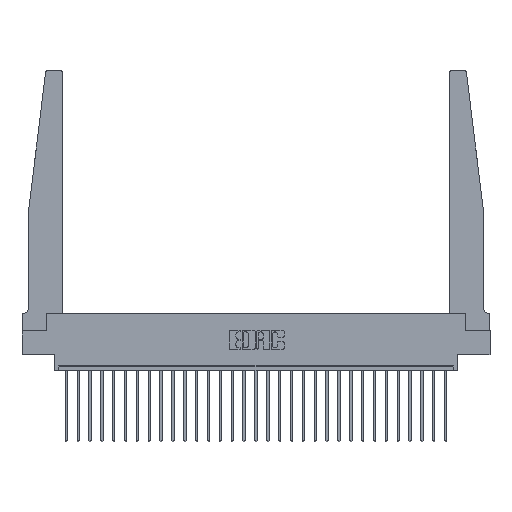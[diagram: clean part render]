
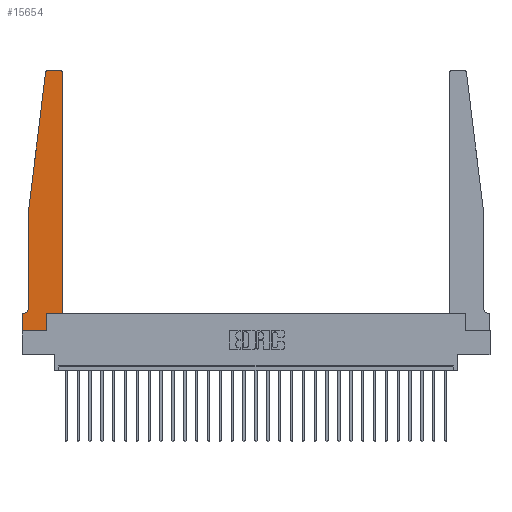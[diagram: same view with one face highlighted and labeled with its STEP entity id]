
A CAD part, top view. The second image highlights one B-rep face of the part: STEP entity #15654.
In plain terms, the highlighted planar face has unit normal (0, 0, 1).
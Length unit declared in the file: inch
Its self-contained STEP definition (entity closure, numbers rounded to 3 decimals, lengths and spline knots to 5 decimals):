
#94 = PLANE ( 'NONE',  #24417 ) ;
#409 = EDGE_CURVE ( 'NONE', #18745, #23858, #8592, .T. ) ;
#501 = FACE_OUTER_BOUND ( 'NONE', #9864, .T. ) ;
#542 = DIRECTION ( 'NONE',  ( 0., -1., 0. ) ) ;
#638 = DIRECTION ( 'NONE',  ( 0., 0., 1. ) ) ;
#757 = DIRECTION ( 'NONE',  ( 1., 0., 0. ) ) ;
#871 = ORIENTED_EDGE ( 'NONE', *, *, #1963, .T. ) ;
#1833 = CARTESIAN_POINT ( 'NONE',  ( 0.065, 1.25, 0.37 ) ) ;
#1963 = EDGE_CURVE ( 'NONE', #26118, #13736, #11295, .T. ) ;
#2018 = EDGE_CURVE ( 'NONE', #22746, #6030, #4937, .T. ) ;
#2330 = LINE ( 'NONE', #15729, #26137 ) ;
#2404 = CARTESIAN_POINT ( 'NONE',  ( 0.2605, 0., 0.37 ) ) ;
#2474 = VERTEX_POINT ( 'NONE', #15890 ) ;
#3025 = VECTOR ( 'NONE', #5932, 39.37008 ) ;
#3362 = DIRECTION ( 'NONE',  ( 0., -1., 0. ) ) ;
#3741 = LINE ( 'NONE', #1833, #3025 ) ;
#4173 = EDGE_CURVE ( 'NONE', #18640, #22746, #21255, .T. ) ;
#4175 = VECTOR ( 'NONE', #26727, 39.37008 ) ;
#4260 = CARTESIAN_POINT ( 'NONE',  ( 0., 0., 0.37 ) ) ;
#4937 = CIRCLE ( 'NONE', #12802, 0.03 ) ;
#5266 = CARTESIAN_POINT ( 'NONE',  ( 0.2605, 0.18, 0.37 ) ) ;
#5402 = DIRECTION ( 'NONE',  ( 0., 0., 1. ) ) ;
#5540 = CARTESIAN_POINT ( 'NONE',  ( 0.27653, 2.75, 0.37 ) ) ;
#5932 = DIRECTION ( 'NONE',  ( -0.122, -0.992, 0. ) ) ;
#6030 = VERTEX_POINT ( 'NONE', #24478 ) ;
#6994 = EDGE_CURVE ( 'NONE', #23858, #26118, #21126, .T. ) ;
#7120 = ORIENTED_EDGE ( 'NONE', *, *, #4173, .T. ) ;
#7160 = ORIENTED_EDGE ( 'NONE', *, *, #13693, .T. ) ;
#7678 = VERTEX_POINT ( 'NONE', #20945 ) ;
#8154 = CARTESIAN_POINT ( 'NONE',  ( 0., 0.1875, 0.37 ) ) ;
#8449 = VERTEX_POINT ( 'NONE', #23913 ) ;
#8592 = LINE ( 'NONE', #10913, #20024 ) ;
#8772 = VECTOR ( 'NONE', #15889, 39.37008 ) ;
#9738 = EDGE_CURVE ( 'NONE', #6030, #22397, #13886, .T. ) ;
#9827 = ORIENTED_EDGE ( 'NONE', *, *, #2018, .T. ) ;
#9864 = EDGE_LOOP ( 'NONE', ( #15268, #23553, #20595, #22302, #7160, #11488, #15987, #17812, #871, #10777, #7120, #9827 ) ) ;
#10184 = EDGE_CURVE ( 'NONE', #22397, #17211, #15628, .T. ) ;
#10320 = VECTOR ( 'NONE', #13755, 39.37008 ) ;
#10777 = ORIENTED_EDGE ( 'NONE', *, *, #18175, .T. ) ;
#10913 = CARTESIAN_POINT ( 'NONE',  ( 0., 0., 0.37 ) ) ;
#10933 = EDGE_CURVE ( 'NONE', #8449, #18745, #2330, .T. ) ;
#11295 = LINE ( 'NONE', #5266, #21563 ) ;
#11404 = DIRECTION ( 'NONE',  ( 0., 0., 1. ) ) ;
#11488 = ORIENTED_EDGE ( 'NONE', *, *, #10933, .T. ) ;
#11969 = LINE ( 'NONE', #18025, #13294 ) ;
#12431 = CARTESIAN_POINT ( 'NONE',  ( 0.015, 0.2375, 0.37 ) ) ;
#12802 = AXIS2_PLACEMENT_3D ( 'NONE', #26090, #5402, #15284 ) ;
#12841 = CARTESIAN_POINT ( 'NONE',  ( 0.2605, 0.18, 0.37 ) ) ;
#13294 = VECTOR ( 'NONE', #3362, 39.37008 ) ;
#13361 = CARTESIAN_POINT ( 'NONE',  ( 0.25, 2.75, 0.37 ) ) ;
#13609 = CARTESIAN_POINT ( 'NONE',  ( 0.24675, 2.72367, 0.37 ) ) ;
#13693 = EDGE_CURVE ( 'NONE', #2474, #8449, #18365, .T. ) ;
#13736 = VERTEX_POINT ( 'NONE', #12841 ) ;
#13755 = DIRECTION ( 'NONE',  ( -1., 0., 0. ) ) ;
#13886 = LINE ( 'NONE', #13361, #10320 ) ;
#14739 = CARTESIAN_POINT ( 'NONE',  ( 0.425, 0.18, 0.37 ) ) ;
#15268 = ORIENTED_EDGE ( 'NONE', *, *, #9738, .T. ) ;
#15284 = DIRECTION ( 'NONE',  ( 1., 0., 0. ) ) ;
#15398 = CARTESIAN_POINT ( 'NONE',  ( 0.27653, 2.72, 0.37 ) ) ;
#15628 = CIRCLE ( 'NONE', #22170, 0.03 ) ;
#15654 = ADVANCED_FACE ( 'NONE', ( #501 ), #94, .T. ) ;
#15729 = CARTESIAN_POINT ( 'NONE',  ( 0.065, 0.1875, 0.37 ) ) ;
#15889 = DIRECTION ( 'NONE',  ( 1., 0., 0. ) ) ;
#15890 = CARTESIAN_POINT ( 'NONE',  ( 0.065, 0.2375, 0.37 ) ) ;
#15959 = EDGE_CURVE ( 'NONE', #17211, #7678, #3741, .T. ) ;
#15987 = ORIENTED_EDGE ( 'NONE', *, *, #409, .T. ) ;
#16226 = CARTESIAN_POINT ( 'NONE',  ( 0.425, 0.18, 0.37 ) ) ;
#16922 = DIRECTION ( 'NONE',  ( 1., 0., 0. ) ) ;
#17211 = VERTEX_POINT ( 'NONE', #13609 ) ;
#17701 = CARTESIAN_POINT ( 'NONE',  ( 0., 0., 0.37 ) ) ;
#17812 = ORIENTED_EDGE ( 'NONE', *, *, #6994, .T. ) ;
#18025 = CARTESIAN_POINT ( 'NONE',  ( 0.065, 1.25, 0.37 ) ) ;
#18175 = EDGE_CURVE ( 'NONE', #13736, #18640, #26285, .T. ) ;
#18258 = CARTESIAN_POINT ( 'NONE',  ( 0.425, 2.72, 0.37 ) ) ;
#18365 = CIRCLE ( 'NONE', #21430, 0.05 ) ;
#18483 = DIRECTION ( 'NONE',  ( -1., 0., 0. ) ) ;
#18526 = VECTOR ( 'NONE', #23437, 39.37008 ) ;
#18640 = VERTEX_POINT ( 'NONE', #14739 ) ;
#18745 = VERTEX_POINT ( 'NONE', #8154 ) ;
#20024 = VECTOR ( 'NONE', #542, 39.37008 ) ;
#20595 = ORIENTED_EDGE ( 'NONE', *, *, #15959, .T. ) ;
#20807 = DIRECTION ( 'NONE',  ( 0., 0., -1. ) ) ;
#20945 = CARTESIAN_POINT ( 'NONE',  ( 0.065, 1.25, 0.37 ) ) ;
#21126 = LINE ( 'NONE', #4260, #4175 ) ;
#21255 = LINE ( 'NONE', #16226, #18526 ) ;
#21430 = AXIS2_PLACEMENT_3D ( 'NONE', #12431, #20807, #18483 ) ;
#21563 = VECTOR ( 'NONE', #21717, 39.37008 ) ;
#21717 = DIRECTION ( 'NONE',  ( 0., 1., 0. ) ) ;
#22170 = AXIS2_PLACEMENT_3D ( 'NONE', #15398, #11404, #757 ) ;
#22302 = ORIENTED_EDGE ( 'NONE', *, *, #23599, .T. ) ;
#22397 = VERTEX_POINT ( 'NONE', #5540 ) ;
#22746 = VERTEX_POINT ( 'NONE', #18258 ) ;
#23437 = DIRECTION ( 'NONE',  ( 0., 1., 0. ) ) ;
#23553 = ORIENTED_EDGE ( 'NONE', *, *, #10184, .T. ) ;
#23599 = EDGE_CURVE ( 'NONE', #7678, #2474, #11969, .T. ) ;
#23858 = VERTEX_POINT ( 'NONE', #17701 ) ;
#23913 = CARTESIAN_POINT ( 'NONE',  ( 0.015, 0.1875, 0.37 ) ) ;
#24082 = DIRECTION ( 'NONE',  ( -1., 0., 0. ) ) ;
#24417 = AXIS2_PLACEMENT_3D ( 'NONE', #25410, #638, #16922 ) ;
#24478 = CARTESIAN_POINT ( 'NONE',  ( 0.395, 2.75, 0.37 ) ) ;
#25410 = CARTESIAN_POINT ( 'NONE',  ( 0., 0.1875, 0.37 ) ) ;
#26090 = CARTESIAN_POINT ( 'NONE',  ( 0.395, 2.72, 0.37 ) ) ;
#26118 = VERTEX_POINT ( 'NONE', #2404 ) ;
#26137 = VECTOR ( 'NONE', #24082, 39.37008 ) ;
#26285 = LINE ( 'NONE', #26426, #8772 ) ;
#26426 = CARTESIAN_POINT ( 'NONE',  ( 0.425, 0.18, 0.37 ) ) ;
#26727 = DIRECTION ( 'NONE',  ( 1., 0., 0. ) ) ;
